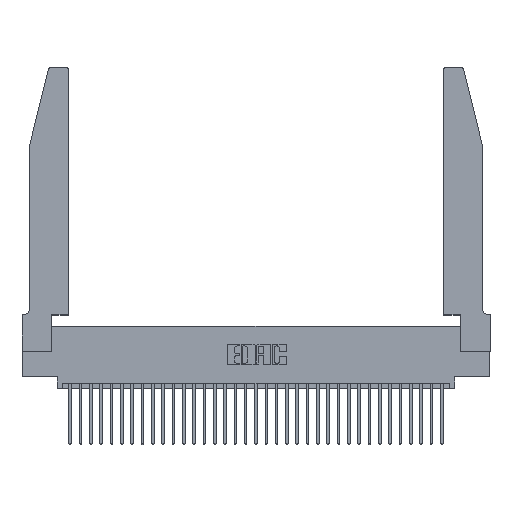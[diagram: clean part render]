
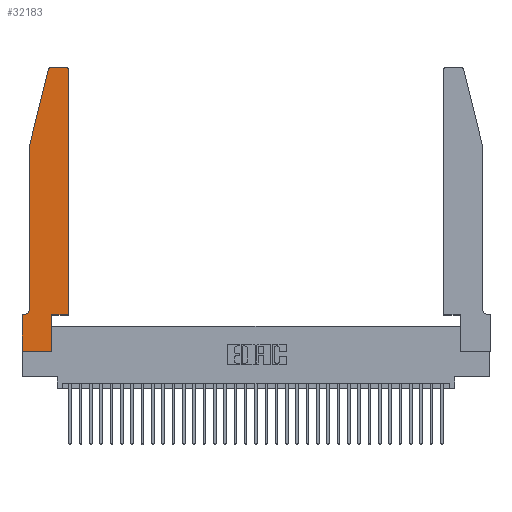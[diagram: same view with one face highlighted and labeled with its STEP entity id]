
A CAD part, top view. The second image highlights one B-rep face of the part: STEP entity #32183.
In plain terms, the highlighted planar face has unit normal (0, 0, 1).
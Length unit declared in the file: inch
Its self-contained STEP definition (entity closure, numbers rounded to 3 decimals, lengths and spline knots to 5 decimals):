
#927 = VERTEX_POINT ( 'NONE', #5334 ) ;
#1000 = CARTESIAN_POINT ( 'NONE',  ( 0.4205, 2.75, 0.37 ) ) ;
#1474 = EDGE_LOOP ( 'NONE', ( #17537, #5854, #16314, #30844, #32908, #13062, #2893, #33740, #10978, #16833, #28040, #22675 ) ) ;
#2086 = VECTOR ( 'NONE', #4153, 39.37008 ) ;
#2289 = DIRECTION ( 'NONE',  ( 0., 0., 1. ) ) ;
#2315 = VERTEX_POINT ( 'NONE', #4909 ) ;
#2476 = EDGE_CURVE ( 'NONE', #2315, #927, #9135, .T. ) ;
#2883 = VECTOR ( 'NONE', #11368, 39.37008 ) ;
#2893 = ORIENTED_EDGE ( 'NONE', *, *, #2476, .T. ) ;
#2969 = LINE ( 'NONE', #30454, #17274 ) ;
#3575 = AXIS2_PLACEMENT_3D ( 'NONE', #8521, #11227, #29797 ) ;
#4153 = DIRECTION ( 'NONE',  ( 0., 1., 0. ) ) ;
#4800 = CARTESIAN_POINT ( 'NONE',  ( 0.284, 2.75, 0.37 ) ) ;
#4909 = CARTESIAN_POINT ( 'NONE',  ( 0., 0.35, 0.37 ) ) ;
#5334 = CARTESIAN_POINT ( 'NONE',  ( 0., 0., 0.37 ) ) ;
#5393 = EDGE_CURVE ( 'NONE', #31928, #26967, #21173, .T. ) ;
#5656 = VERTEX_POINT ( 'NONE', #28216 ) ;
#5854 = ORIENTED_EDGE ( 'NONE', *, *, #25293, .T. ) ;
#5983 = VECTOR ( 'NONE', #31346, 39.37008 ) ;
#6395 = EDGE_CURVE ( 'NONE', #927, #18250, #11526, .T. ) ;
#6857 = CARTESIAN_POINT ( 'NONE',  ( 0.4505, 0.35, 0.37 ) ) ;
#7699 = EDGE_CURVE ( 'NONE', #18250, #13058, #13132, .T. ) ;
#8294 = VECTOR ( 'NONE', #26706, 39.37008 ) ;
#8512 = CARTESIAN_POINT ( 'NONE',  ( 0.0055, 0.35, 0.37 ) ) ;
#8521 = CARTESIAN_POINT ( 'NONE',  ( 0., 0.35, 0.37 ) ) ;
#9135 = LINE ( 'NONE', #18827, #8294 ) ;
#9251 = LINE ( 'NONE', #27246, #2883 ) ;
#10481 = CIRCLE ( 'NONE', #18171, 0.03 ) ;
#10872 = VERTEX_POINT ( 'NONE', #31650 ) ;
#10978 = ORIENTED_EDGE ( 'NONE', *, *, #7699, .T. ) ;
#11227 = DIRECTION ( 'NONE',  ( 0., 0., 1. ) ) ;
#11290 = EDGE_CURVE ( 'NONE', #10872, #19415, #30706, .T. ) ;
#11294 = CARTESIAN_POINT ( 'NONE',  ( 0.0055, 0.42, 0.37 ) ) ;
#11368 = DIRECTION ( 'NONE',  ( 0., -1., 0. ) ) ;
#11526 = LINE ( 'NONE', #12886, #17743 ) ;
#11713 = LINE ( 'NONE', #26534, #32056 ) ;
#12234 = DIRECTION ( 'NONE',  ( 0., 0., 1. ) ) ;
#12886 = CARTESIAN_POINT ( 'NONE',  ( 0., 0., 0.37 ) ) ;
#13058 = VERTEX_POINT ( 'NONE', #22820 ) ;
#13062 = ORIENTED_EDGE ( 'NONE', *, *, #29781, .T. ) ;
#13064 = EDGE_CURVE ( 'NONE', #13058, #5656, #13225, .T. ) ;
#13132 = LINE ( 'NONE', #15472, #5983 ) ;
#13225 = LINE ( 'NONE', #6857, #26477 ) ;
#13341 = DIRECTION ( 'NONE',  ( -1., 0., 0. ) ) ;
#13997 = DIRECTION ( 'NONE',  ( -1., 0., 0. ) ) ;
#14781 = LINE ( 'NONE', #22861, #2086 ) ;
#14946 = DIRECTION ( 'NONE',  ( 1., 0., 0. ) ) ;
#15472 = CARTESIAN_POINT ( 'NONE',  ( 0.2865, 0.35, 0.37 ) ) ;
#16314 = ORIENTED_EDGE ( 'NONE', *, *, #11290, .T. ) ;
#16676 = CARTESIAN_POINT ( 'NONE',  ( 0.0755, 2., 0.37 ) ) ;
#16833 = ORIENTED_EDGE ( 'NONE', *, *, #13064, .T. ) ;
#16845 = EDGE_CURVE ( 'NONE', #16955, #33109, #11713, .T. ) ;
#16955 = VERTEX_POINT ( 'NONE', #1000 ) ;
#17121 = DIRECTION ( 'NONE',  ( -1., 0., 0. ) ) ;
#17274 = VECTOR ( 'NONE', #17121, 39.37008 ) ;
#17537 = ORIENTED_EDGE ( 'NONE', *, *, #16845, .T. ) ;
#17743 = VECTOR ( 'NONE', #20767, 39.37008 ) ;
#18171 = AXIS2_PLACEMENT_3D ( 'NONE', #18376, #2289, #21062 ) ;
#18250 = VERTEX_POINT ( 'NONE', #27389 ) ;
#18376 = CARTESIAN_POINT ( 'NONE',  ( 0.4205, 2.72, 0.37 ) ) ;
#18827 = CARTESIAN_POINT ( 'NONE',  ( 0., 0., 0.37 ) ) ;
#19415 = VERTEX_POINT ( 'NONE', #16676 ) ;
#20767 = DIRECTION ( 'NONE',  ( 1., 0., 0. ) ) ;
#20975 = EDGE_CURVE ( 'NONE', #5656, #23778, #14781, .T. ) ;
#21062 = DIRECTION ( 'NONE',  ( 1., 0., 0. ) ) ;
#21164 = CIRCLE ( 'NONE', #30056, 0.03 ) ;
#21169 = CARTESIAN_POINT ( 'NONE',  ( 0.4505, 2.72, 0.37 ) ) ;
#21173 = CIRCLE ( 'NONE', #29429, 0.07 ) ;
#21692 = FACE_OUTER_BOUND ( 'NONE', #1474, .T. ) ;
#22547 = EDGE_CURVE ( 'NONE', #19415, #31928, #9251, .T. ) ;
#22675 = ORIENTED_EDGE ( 'NONE', *, *, #31426, .T. ) ;
#22820 = CARTESIAN_POINT ( 'NONE',  ( 0.2865, 0.35, 0.37 ) ) ;
#22861 = CARTESIAN_POINT ( 'NONE',  ( 0.4505, 0.35, 0.37 ) ) ;
#23778 = VERTEX_POINT ( 'NONE', #21169 ) ;
#24479 = PLANE ( 'NONE',  #3575 ) ;
#25293 = EDGE_CURVE ( 'NONE', #33109, #10872, #21164, .T. ) ;
#26146 = DIRECTION ( 'NONE',  ( -0.239, -0.971, 0. ) ) ;
#26477 = VECTOR ( 'NONE', #14946, 39.37008 ) ;
#26534 = CARTESIAN_POINT ( 'NONE',  ( 0.2605, 2.75, 0.37 ) ) ;
#26706 = DIRECTION ( 'NONE',  ( 0., -1., 0. ) ) ;
#26967 = VERTEX_POINT ( 'NONE', #8512 ) ;
#27246 = CARTESIAN_POINT ( 'NONE',  ( 0.0755, 2., 0.37 ) ) ;
#27389 = CARTESIAN_POINT ( 'NONE',  ( 0.2865, 0., 0.37 ) ) ;
#28040 = ORIENTED_EDGE ( 'NONE', *, *, #20975, .T. ) ;
#28114 = CARTESIAN_POINT ( 'NONE',  ( 0.284, 2.72, 0.37 ) ) ;
#28216 = CARTESIAN_POINT ( 'NONE',  ( 0.4505, 0.35, 0.37 ) ) ;
#28683 = CARTESIAN_POINT ( 'NONE',  ( 0.0755, 2., 0.37 ) ) ;
#29429 = AXIS2_PLACEMENT_3D ( 'NONE', #11294, #29857, #13997 ) ;
#29781 = EDGE_CURVE ( 'NONE', #26967, #2315, #2969, .T. ) ;
#29797 = DIRECTION ( 'NONE',  ( 1., 0., 0. ) ) ;
#29853 = VECTOR ( 'NONE', #26146, 39.37008 ) ;
#29857 = DIRECTION ( 'NONE',  ( 0., 0., -1. ) ) ;
#30056 = AXIS2_PLACEMENT_3D ( 'NONE', #28114, #12234, #30797 ) ;
#30454 = CARTESIAN_POINT ( 'NONE',  ( 0.0755, 0.35, 0.37 ) ) ;
#30706 = LINE ( 'NONE', #28683, #29853 ) ;
#30797 = DIRECTION ( 'NONE',  ( 1., 0., 0. ) ) ;
#30844 = ORIENTED_EDGE ( 'NONE', *, *, #22547, .T. ) ;
#31346 = DIRECTION ( 'NONE',  ( 0., 1., 0. ) ) ;
#31426 = EDGE_CURVE ( 'NONE', #23778, #16955, #10481, .T. ) ;
#31650 = CARTESIAN_POINT ( 'NONE',  ( 0.25487, 2.72718, 0.37 ) ) ;
#31928 = VERTEX_POINT ( 'NONE', #33598 ) ;
#32056 = VECTOR ( 'NONE', #13341, 39.37008 ) ;
#32183 = ADVANCED_FACE ( 'NONE', ( #21692 ), #24479, .T. ) ;
#32908 = ORIENTED_EDGE ( 'NONE', *, *, #5393, .T. ) ;
#33109 = VERTEX_POINT ( 'NONE', #4800 ) ;
#33598 = CARTESIAN_POINT ( 'NONE',  ( 0.0755, 0.42, 0.37 ) ) ;
#33740 = ORIENTED_EDGE ( 'NONE', *, *, #6395, .T. ) ;
